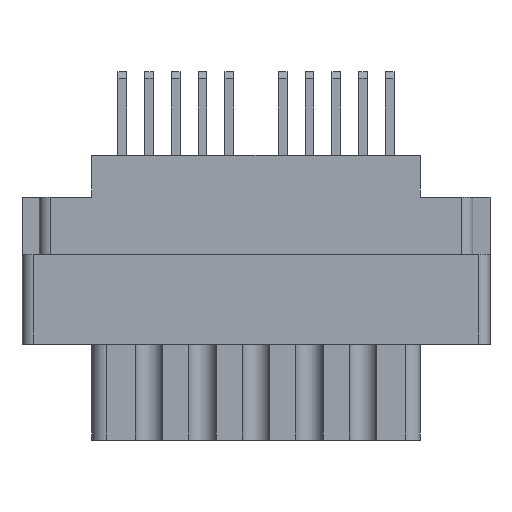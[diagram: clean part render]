
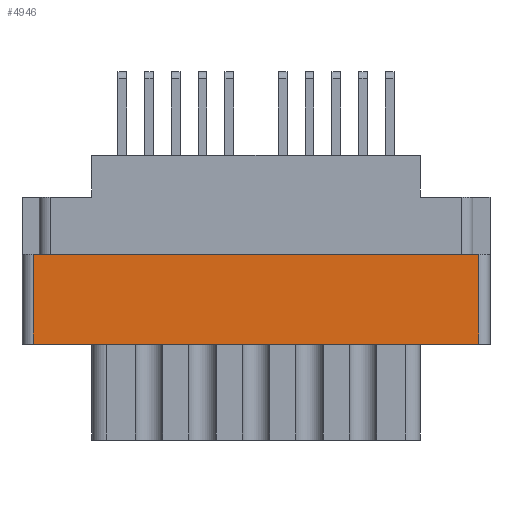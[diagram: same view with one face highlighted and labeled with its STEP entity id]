
A CAD part, front view. The second image highlights one B-rep face of the part: STEP entity #4946.
In plain terms, the highlighted planar face has unit normal (0, -1, 0).
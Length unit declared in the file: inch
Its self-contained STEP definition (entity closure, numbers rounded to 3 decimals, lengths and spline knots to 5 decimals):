
#1763 = CARTESIAN_POINT ( 'NONE',  ( 0., -0.343, -0.529 ) ) ;
#2134 = ORIENTED_EDGE ( 'NONE', *, *, #5999, .T. ) ;
#2470 = FACE_OUTER_BOUND ( 'NONE', #22843, .T. ) ;
#2829 = VERTEX_POINT ( 'NONE', #4399 ) ;
#3400 = CARTESIAN_POINT ( 'NONE',  ( -0.624, -0.343, -0.798 ) ) ;
#3859 = VECTOR ( 'NONE', #13004, 39.37008 ) ;
#4399 = CARTESIAN_POINT ( 'NONE',  ( -0.624, -0.343, -0.529 ) ) ;
#4848 = ORIENTED_EDGE ( 'NONE', *, *, #22907, .F. ) ;
#4946 = ADVANCED_FACE ( 'NONE', ( #2470 ), #11641, .T. ) ;
#5374 = DIRECTION ( 'NONE',  ( -1., 0., 0. ) ) ;
#5999 = EDGE_CURVE ( 'NONE', #17054, #10293, #14304, .T. ) ;
#6356 = LINE ( 'NONE', #1763, #11875 ) ;
#7568 = CARTESIAN_POINT ( 'NONE',  ( 0.624, -0.343, -0.798 ) ) ;
#8030 = ORIENTED_EDGE ( 'NONE', *, *, #12151, .T. ) ;
#8174 = LINE ( 'NONE', #20864, #16901 ) ;
#9106 = VERTEX_POINT ( 'NONE', #14986 ) ;
#10293 = VERTEX_POINT ( 'NONE', #18739 ) ;
#10638 = DIRECTION ( 'NONE',  ( 1., 0., 0. ) ) ;
#10681 = EDGE_CURVE ( 'NONE', #17054, #2829, #6356, .T. ) ;
#11641 = PLANE ( 'NONE',  #20235 ) ;
#11875 = VECTOR ( 'NONE', #5374, 39.37008 ) ;
#11899 = CARTESIAN_POINT ( 'NONE',  ( -0.656, -0.343, -0.798 ) ) ;
#12151 = EDGE_CURVE ( 'NONE', #9106, #2829, #23138, .T. ) ;
#12704 = ORIENTED_EDGE ( 'NONE', *, *, #10681, .F. ) ;
#13004 = DIRECTION ( 'NONE',  ( 0., 0., 1. ) ) ;
#13513 = DIRECTION ( 'NONE',  ( 0., -1., 0. ) ) ;
#13760 = DIRECTION ( 'NONE',  ( 0., 0., -1. ) ) ;
#14304 = LINE ( 'NONE', #7568, #3859 ) ;
#14986 = CARTESIAN_POINT ( 'NONE',  ( -0.624, -0.343, -0.277 ) ) ;
#16901 = VECTOR ( 'NONE', #10638, 39.37008 ) ;
#17054 = VERTEX_POINT ( 'NONE', #23400 ) ;
#18474 = DIRECTION ( 'NONE',  ( 0., 0., -1. ) ) ;
#18739 = CARTESIAN_POINT ( 'NONE',  ( 0.624, -0.343, -0.277 ) ) ;
#20235 = AXIS2_PLACEMENT_3D ( 'NONE', #11899, #13513, #13760 ) ;
#20864 = CARTESIAN_POINT ( 'NONE',  ( 0., -0.343, -0.277 ) ) ;
#22558 = VECTOR ( 'NONE', #18474, 39.37008 ) ;
#22843 = EDGE_LOOP ( 'NONE', ( #4848, #8030, #12704, #2134 ) ) ;
#22907 = EDGE_CURVE ( 'NONE', #9106, #10293, #8174, .T. ) ;
#23138 = LINE ( 'NONE', #3400, #22558 ) ;
#23400 = CARTESIAN_POINT ( 'NONE',  ( 0.624, -0.343, -0.529 ) ) ;
